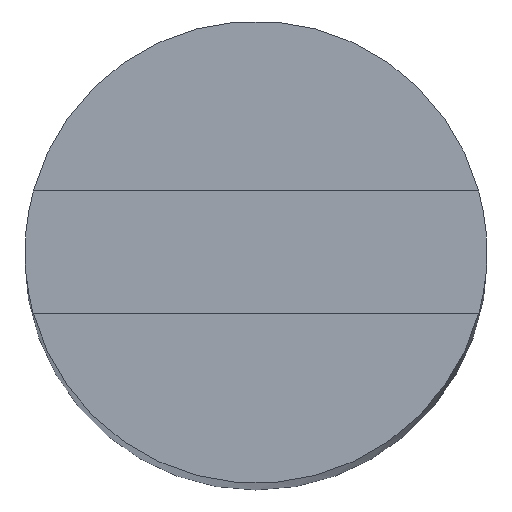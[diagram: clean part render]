
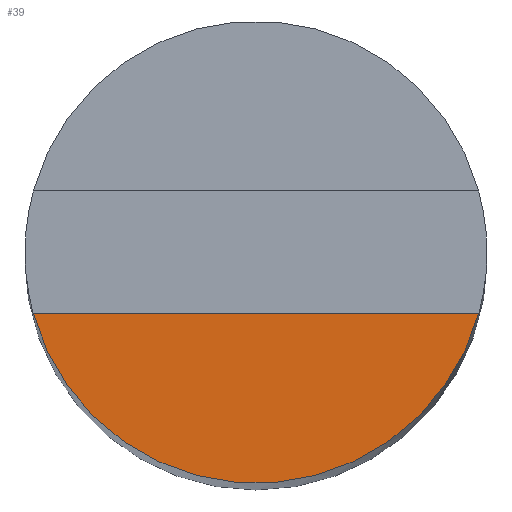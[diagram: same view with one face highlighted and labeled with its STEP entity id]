
A CAD part, top view. The second image highlights one B-rep face of the part: STEP entity #39.
In plain terms, the highlighted planar face has unit normal (0, 0, 1).
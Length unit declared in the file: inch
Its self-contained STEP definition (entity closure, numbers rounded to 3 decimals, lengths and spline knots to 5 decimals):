
#2 = VERTEX_POINT ( 'NONE', #66 ) ;
#14 = AXIS2_PLACEMENT_3D ( 'NONE', #323, #172, #302 ) ;
#15 = VECTOR ( 'NONE', #153, 39.37008 ) ;
#24 = CARTESIAN_POINT ( 'NONE',  ( 0., -0.0125, 0.45 ) ) ;
#38 = AXIS2_PLACEMENT_3D ( 'NONE', #204, #290, #104 ) ;
#39 = ADVANCED_FACE ( 'NONE', ( #327 ), #75, .T. ) ;
#50 = ORIENTED_EDGE ( 'NONE', *, *, #110, .F. ) ;
#56 = VERTEX_POINT ( 'NONE', #182 ) ;
#66 = CARTESIAN_POINT ( 'NONE',  ( 0.0452, -0.0125, 0.45 ) ) ;
#75 = PLANE ( 'NONE',  #38 ) ;
#93 = EDGE_CURVE ( 'NONE', #56, #2, #137, .T. ) ;
#104 = DIRECTION ( 'NONE',  ( 1., 0., 0. ) ) ;
#110 = EDGE_CURVE ( 'NONE', #56, #2, #227, .T. ) ;
#137 = CIRCLE ( 'NONE', #14, 0.0469 ) ;
#148 = EDGE_LOOP ( 'NONE', ( #50, #305 ) ) ;
#153 = DIRECTION ( 'NONE',  ( 1., 0., 0. ) ) ;
#172 = DIRECTION ( 'NONE',  ( 0., 0., 1. ) ) ;
#182 = CARTESIAN_POINT ( 'NONE',  ( -0.0452, -0.0125, 0.45 ) ) ;
#204 = CARTESIAN_POINT ( 'NONE',  ( 0., 0., 0.45 ) ) ;
#227 = LINE ( 'NONE', #24, #15 ) ;
#290 = DIRECTION ( 'NONE',  ( 0., 0., 1. ) ) ;
#302 = DIRECTION ( 'NONE',  ( 1., 0., 0. ) ) ;
#305 = ORIENTED_EDGE ( 'NONE', *, *, #93, .T. ) ;
#323 = CARTESIAN_POINT ( 'NONE',  ( 0., 0., 0.45 ) ) ;
#327 = FACE_OUTER_BOUND ( 'NONE', #148, .T. ) ;
